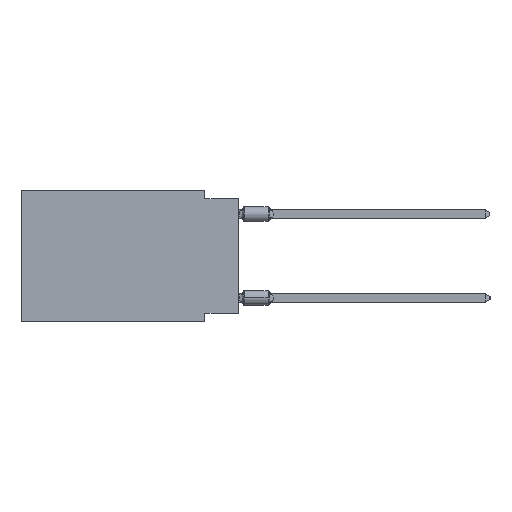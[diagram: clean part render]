
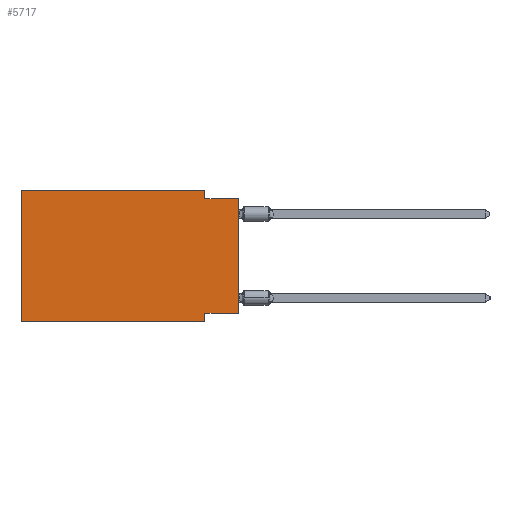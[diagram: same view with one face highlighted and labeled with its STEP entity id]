
A CAD part, left-side view. The second image highlights one B-rep face of the part: STEP entity #5717.
In plain terms, the highlighted planar face has unit normal (-1, 0, 0).
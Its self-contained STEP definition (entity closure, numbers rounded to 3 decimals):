
#1424 = EDGE_CURVE ( 'NONE', #37447, #50127, #16562, .T. ) ;
#3004 = VERTEX_POINT ( 'NONE', #10859 ) ;
#3423 = VECTOR ( 'NONE', #12499, 1000. ) ;
#3623 = LINE ( 'NONE', #33431, #25636 ) ;
#3838 = FACE_OUTER_BOUND ( 'NONE', #7788, .T. ) ;
#5717 = ADVANCED_FACE ( 'NONE', ( #3838 ), #36641, .F. ) ;
#7788 = EDGE_LOOP ( 'NONE', ( #17103, #14821, #19556, #34066, #21090, #40599, #47151, #24563 ) ) ;
#8901 = VECTOR ( 'NONE', #9961, 1000. ) ;
#9961 = DIRECTION ( 'NONE',  ( 0., 0., -1. ) ) ;
#10134 = EDGE_CURVE ( 'NONE', #47969, #17950, #30299, .T. ) ;
#10178 = VERTEX_POINT ( 'NONE', #21898 ) ;
#10859 = CARTESIAN_POINT ( 'NONE',  ( 0., 16.383, -9.906 ) ) ;
#11002 = VERTEX_POINT ( 'NONE', #35246 ) ;
#11048 = EDGE_CURVE ( 'NONE', #50127, #11002, #51249, .T. ) ;
#11248 = DIRECTION ( 'NONE',  ( 0., 0., 1. ) ) ;
#12007 = EDGE_CURVE ( 'NONE', #3004, #28813, #32135, .T. ) ;
#12499 = DIRECTION ( 'NONE',  ( 0., 1., 0. ) ) ;
#14821 = ORIENTED_EDGE ( 'NONE', *, *, #33324, .F. ) ;
#14862 = EDGE_CURVE ( 'NONE', #37447, #10178, #37954, .T. ) ;
#15154 = CARTESIAN_POINT ( 'NONE',  ( 0., 2.54, 0. ) ) ;
#16043 = DIRECTION ( 'NONE',  ( 1., 0., 0. ) ) ;
#16562 = LINE ( 'NONE', #29280, #3423 ) ;
#17103 = ORIENTED_EDGE ( 'NONE', *, *, #14862, .T. ) ;
#17950 = VERTEX_POINT ( 'NONE', #39619 ) ;
#19556 = ORIENTED_EDGE ( 'NONE', *, *, #10134, .F. ) ;
#19697 = CARTESIAN_POINT ( 'NONE',  ( 0., 0., -9.271 ) ) ;
#19951 = VECTOR ( 'NONE', #11248, 1000. ) ;
#21090 = ORIENTED_EDGE ( 'NONE', *, *, #12007, .F. ) ;
#21532 = CARTESIAN_POINT ( 'NONE',  ( 0., 0., -0.635 ) ) ;
#21898 = CARTESIAN_POINT ( 'NONE',  ( 0., 0., -0.635 ) ) ;
#22641 = CARTESIAN_POINT ( 'NONE',  ( 0., 2.54, -9.271 ) ) ;
#24563 = ORIENTED_EDGE ( 'NONE', *, *, #1424, .F. ) ;
#24998 = VECTOR ( 'NONE', #41503, 1000. ) ;
#25636 = VECTOR ( 'NONE', #32647, 1000. ) ;
#28813 = VERTEX_POINT ( 'NONE', #40589 ) ;
#29280 = CARTESIAN_POINT ( 'NONE',  ( 0., 0., -9.271 ) ) ;
#29660 = LINE ( 'NONE', #21532, #33292 ) ;
#30299 = LINE ( 'NONE', #47101, #8901 ) ;
#31184 = CARTESIAN_POINT ( 'NONE',  ( 0., 2.54, -9.906 ) ) ;
#32135 = LINE ( 'NONE', #35929, #19951 ) ;
#32647 = DIRECTION ( 'NONE',  ( 0., -1., 0. ) ) ;
#33292 = VECTOR ( 'NONE', #38066, 1000. ) ;
#33324 = EDGE_CURVE ( 'NONE', #17950, #10178, #29660, .T. ) ;
#33431 = CARTESIAN_POINT ( 'NONE',  ( 0., 16.383, -9.906 ) ) ;
#33757 = VECTOR ( 'NONE', #34426, 1000. ) ;
#33898 = CARTESIAN_POINT ( 'NONE',  ( 0., 0., 0. ) ) ;
#34066 = ORIENTED_EDGE ( 'NONE', *, *, #49361, .F. ) ;
#34267 = VECTOR ( 'NONE', #52838, 1000. ) ;
#34426 = DIRECTION ( 'NONE',  ( 0., 0., -1. ) ) ;
#35246 = CARTESIAN_POINT ( 'NONE',  ( 0., 2.54, -9.906 ) ) ;
#35929 = CARTESIAN_POINT ( 'NONE',  ( 0., 16.383, 0. ) ) ;
#36286 = LINE ( 'NONE', #49030, #34267 ) ;
#36641 = PLANE ( 'NONE',  #47821 ) ;
#37447 = VERTEX_POINT ( 'NONE', #19697 ) ;
#37954 = LINE ( 'NONE', #33898, #24998 ) ;
#38066 = DIRECTION ( 'NONE',  ( 0., -1., 0. ) ) ;
#39619 = CARTESIAN_POINT ( 'NONE',  ( 0., 2.54, -0.635 ) ) ;
#40589 = CARTESIAN_POINT ( 'NONE',  ( 0., 16.383, 0. ) ) ;
#40599 = ORIENTED_EDGE ( 'NONE', *, *, #51408, .T. ) ;
#41503 = DIRECTION ( 'NONE',  ( 0., 0., 1. ) ) ;
#47101 = CARTESIAN_POINT ( 'NONE',  ( 0., 2.54, 0. ) ) ;
#47151 = ORIENTED_EDGE ( 'NONE', *, *, #11048, .F. ) ;
#47821 = AXIS2_PLACEMENT_3D ( 'NONE', #53201, #16043, #53451 ) ;
#47969 = VERTEX_POINT ( 'NONE', #15154 ) ;
#49030 = CARTESIAN_POINT ( 'NONE',  ( 0., 16.383, 0. ) ) ;
#49361 = EDGE_CURVE ( 'NONE', #28813, #47969, #36286, .T. ) ;
#50127 = VERTEX_POINT ( 'NONE', #22641 ) ;
#51249 = LINE ( 'NONE', #31184, #33757 ) ;
#51408 = EDGE_CURVE ( 'NONE', #3004, #11002, #3623, .T. ) ;
#52838 = DIRECTION ( 'NONE',  ( 0., -1., 0. ) ) ;
#53201 = CARTESIAN_POINT ( 'NONE',  ( 0., 16.383, 0. ) ) ;
#53451 = DIRECTION ( 'NONE',  ( 0., 0., -1. ) ) ;
